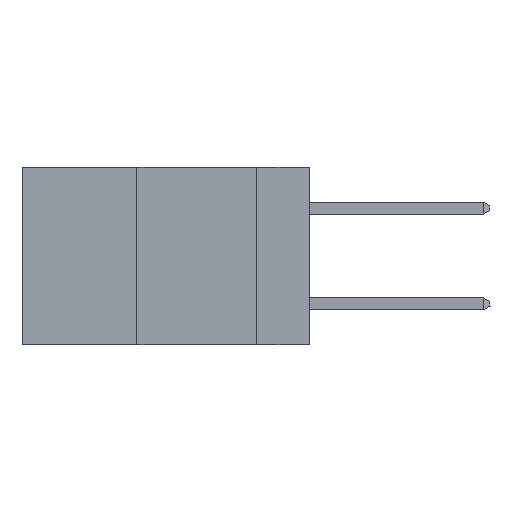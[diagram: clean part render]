
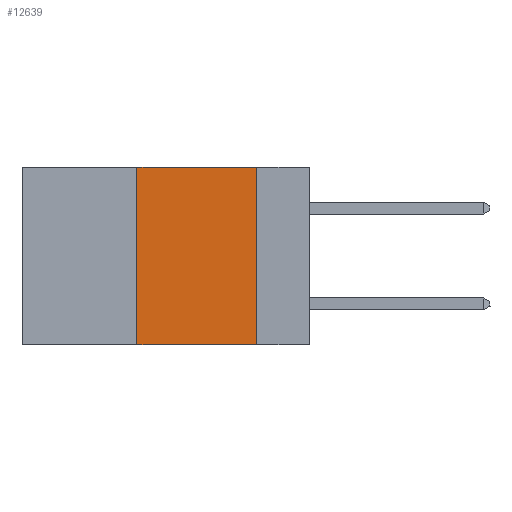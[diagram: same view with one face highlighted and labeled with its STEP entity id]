
A CAD part, left-side view. The second image highlights one B-rep face of the part: STEP entity #12639.
In plain terms, the highlighted planar face has unit normal (-1, 0, 0).
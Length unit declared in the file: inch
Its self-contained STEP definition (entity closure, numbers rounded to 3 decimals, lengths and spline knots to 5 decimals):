
#192 = CARTESIAN_POINT ( 'NONE',  ( 0., 0.6, -0.37 ) ) ;
#391 = ORIENTED_EDGE ( 'NONE', *, *, #5416, .T. ) ;
#555 = CARTESIAN_POINT ( 'NONE',  ( 0., 0.11, 0. ) ) ;
#941 = LINE ( 'NONE', #4571, #9565 ) ;
#1033 = VERTEX_POINT ( 'NONE', #2545 ) ;
#1334 = DIRECTION ( 'NONE',  ( 0., 0., -1. ) ) ;
#1460 = PLANE ( 'NONE',  #11459 ) ;
#1826 = VERTEX_POINT ( 'NONE', #8914 ) ;
#2169 = EDGE_CURVE ( 'NONE', #1033, #7517, #7660, .T. ) ;
#2545 = CARTESIAN_POINT ( 'NONE',  ( 0., 0.36, -0.37 ) ) ;
#2553 = DIRECTION ( 'NONE',  ( 0., 0., -1. ) ) ;
#3000 = ORIENTED_EDGE ( 'NONE', *, *, #6141, .F. ) ;
#4155 = LINE ( 'NONE', #192, #9240 ) ;
#4571 = CARTESIAN_POINT ( 'NONE',  ( 0., 0.11, 0. ) ) ;
#4644 = CARTESIAN_POINT ( 'NONE',  ( 0., 0.6, 0. ) ) ;
#5416 = EDGE_CURVE ( 'NONE', #1033, #1826, #4155, .T. ) ;
#5436 = EDGE_CURVE ( 'NONE', #7762, #1826, #941, .T. ) ;
#6141 = EDGE_CURVE ( 'NONE', #7517, #7762, #11494, .T. ) ;
#6709 = DIRECTION ( 'NONE',  ( 0., -1., 0. ) ) ;
#7345 = VECTOR ( 'NONE', #10477, 39.37008 ) ;
#7517 = VERTEX_POINT ( 'NONE', #11998 ) ;
#7660 = LINE ( 'NONE', #9447, #7345 ) ;
#7762 = VERTEX_POINT ( 'NONE', #555 ) ;
#8125 = ORIENTED_EDGE ( 'NONE', *, *, #5436, .F. ) ;
#8433 = VECTOR ( 'NONE', #6709, 39.37008 ) ;
#8603 = DIRECTION ( 'NONE',  ( 0., -1., 0. ) ) ;
#8678 = CARTESIAN_POINT ( 'NONE',  ( 0., 0.6, 0. ) ) ;
#8720 = DIRECTION ( 'NONE',  ( 1., 0., 0. ) ) ;
#8914 = CARTESIAN_POINT ( 'NONE',  ( 0., 0.11, -0.37 ) ) ;
#9240 = VECTOR ( 'NONE', #8603, 39.37008 ) ;
#9447 = CARTESIAN_POINT ( 'NONE',  ( 0., 0.36, 0. ) ) ;
#9565 = VECTOR ( 'NONE', #1334, 39.37008 ) ;
#10477 = DIRECTION ( 'NONE',  ( 0., 0., 1. ) ) ;
#11192 = ORIENTED_EDGE ( 'NONE', *, *, #2169, .F. ) ;
#11459 = AXIS2_PLACEMENT_3D ( 'NONE', #8678, #8720, #2553 ) ;
#11494 = LINE ( 'NONE', #4644, #8433 ) ;
#11998 = CARTESIAN_POINT ( 'NONE',  ( 0., 0.36, 0. ) ) ;
#12000 = FACE_OUTER_BOUND ( 'NONE', #12107, .T. ) ;
#12107 = EDGE_LOOP ( 'NONE', ( #8125, #3000, #11192, #391 ) ) ;
#12639 = ADVANCED_FACE ( 'NONE', ( #12000 ), #1460, .F. ) ;
